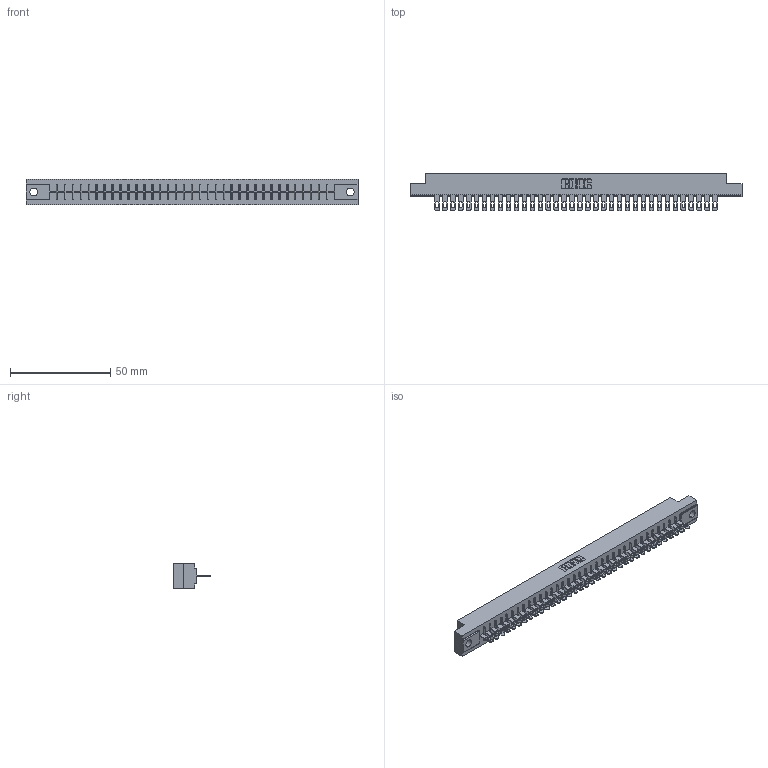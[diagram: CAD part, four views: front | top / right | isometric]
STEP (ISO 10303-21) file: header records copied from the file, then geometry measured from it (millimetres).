
FILE_DESCRIPTION (( 'STEP AP203' ), '1' );
FILE_NAME ('306-036-500-104.STEP', '2019-09-11T23:28:06', ( '' ), ( '' ), 'SwSTEP 2.0', 'SolidWorks 2016', '' );
FILE_SCHEMA (( 'CONFIG_CONTROL_DESIGN' ));
Length unit declared in the file: inch
Products named in the file (3): 306-290-001_100; 306-036-500-104; 306 Part_.156 Dia
Assembly tree (37 placements, depth 2):
  306-036-500-104
    306 Part_.156 Dia
    306-290-001_100  x36
Bounding box: 165.66 x 18.87 x 12.7 mm (x, y, z)
Volume: 18273.8 mm3; surface area: 19145.4 mm2
Topology: 37 solids, 37 shells, 2866 faces, 8092 edges, 5200 vertices
Faces by surface type: plane 1882, cylinder 840, sphere 144
Entity records: 34931 total; most frequent: CARTESIAN_POINT 5869, ORIENTED_EDGE 5816, DIRECTION 5780, EDGE_CURVE 2908, VECTOR 2278, LINE 2278, VERTEX_POINT 1840, AXIS2_PLACEMENT_3D 1751
